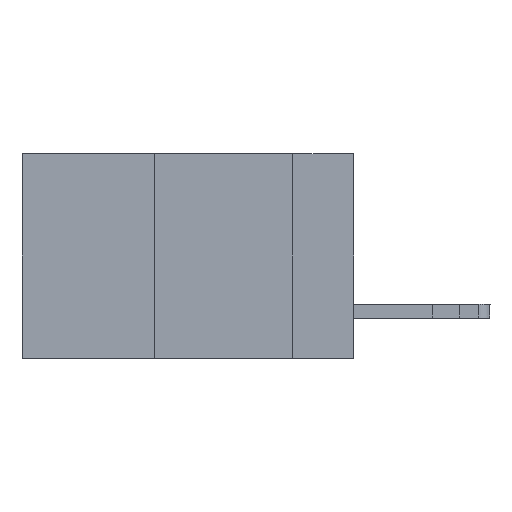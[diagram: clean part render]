
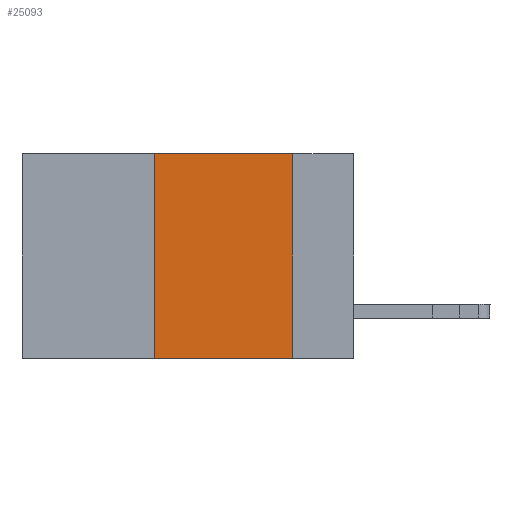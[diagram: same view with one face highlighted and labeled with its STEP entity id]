
A CAD part, left-side view. The second image highlights one B-rep face of the part: STEP entity #25093.
In plain terms, the highlighted planar face has unit normal (-1, 0, 0).
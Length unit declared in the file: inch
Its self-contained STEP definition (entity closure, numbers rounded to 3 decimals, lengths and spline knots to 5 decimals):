
#22 = EDGE_CURVE ( 'NONE', #27351, #13392, #2701, .T. ) ;
#625 = LINE ( 'NONE', #28062, #6468 ) ;
#1461 = ORIENTED_EDGE ( 'NONE', *, *, #17476, .F. ) ;
#2701 = LINE ( 'NONE', #22874, #16120 ) ;
#3524 = ORIENTED_EDGE ( 'NONE', *, *, #22, .T. ) ;
#4197 = VERTEX_POINT ( 'NONE', #27617 ) ;
#5993 = CARTESIAN_POINT ( 'NONE',  ( 0., 0.36, -0.37 ) ) ;
#6354 = FACE_OUTER_BOUND ( 'NONE', #8347, .T. ) ;
#6468 = VECTOR ( 'NONE', #9905, 39.37008 ) ;
#6851 = LINE ( 'NONE', #27795, #22669 ) ;
#8347 = EDGE_LOOP ( 'NONE', ( #20347, #28427, #1461, #3524 ) ) ;
#9253 = CARTESIAN_POINT ( 'NONE',  ( 0., 0.11, 0. ) ) ;
#9833 = LINE ( 'NONE', #27833, #21288 ) ;
#9905 = DIRECTION ( 'NONE',  ( 0., 0., -1. ) ) ;
#11380 = DIRECTION ( 'NONE',  ( 0., -1., 0. ) ) ;
#11556 = VERTEX_POINT ( 'NONE', #9253 ) ;
#12836 = PLANE ( 'NONE',  #16813 ) ;
#13106 = CARTESIAN_POINT ( 'NONE',  ( 0., 0.11, -0.37 ) ) ;
#13263 = CARTESIAN_POINT ( 'NONE',  ( 0., 0.6, 0. ) ) ;
#13392 = VERTEX_POINT ( 'NONE', #13106 ) ;
#14508 = DIRECTION ( 'NONE',  ( 0., -1., 0. ) ) ;
#15163 = DIRECTION ( 'NONE',  ( 1., 0., 0. ) ) ;
#16120 = VECTOR ( 'NONE', #11380, 39.37008 ) ;
#16813 = AXIS2_PLACEMENT_3D ( 'NONE', #13263, #15163, #28503 ) ;
#17476 = EDGE_CURVE ( 'NONE', #27351, #4197, #6851, .T. ) ;
#18712 = DIRECTION ( 'NONE',  ( 0., 0., 1. ) ) ;
#18840 = EDGE_CURVE ( 'NONE', #4197, #11556, #9833, .T. ) ;
#20347 = ORIENTED_EDGE ( 'NONE', *, *, #28890, .F. ) ;
#21288 = VECTOR ( 'NONE', #14508, 39.37008 ) ;
#22669 = VECTOR ( 'NONE', #18712, 39.37008 ) ;
#22874 = CARTESIAN_POINT ( 'NONE',  ( 0., 0.6, -0.37 ) ) ;
#25093 = ADVANCED_FACE ( 'NONE', ( #6354 ), #12836, .F. ) ;
#27351 = VERTEX_POINT ( 'NONE', #5993 ) ;
#27617 = CARTESIAN_POINT ( 'NONE',  ( 0., 0.36, 0. ) ) ;
#27795 = CARTESIAN_POINT ( 'NONE',  ( 0., 0.36, 0. ) ) ;
#27833 = CARTESIAN_POINT ( 'NONE',  ( 0., 0.6, 0. ) ) ;
#28062 = CARTESIAN_POINT ( 'NONE',  ( 0., 0.11, 0. ) ) ;
#28427 = ORIENTED_EDGE ( 'NONE', *, *, #18840, .F. ) ;
#28503 = DIRECTION ( 'NONE',  ( 0., 0., -1. ) ) ;
#28890 = EDGE_CURVE ( 'NONE', #11556, #13392, #625, .T. ) ;
